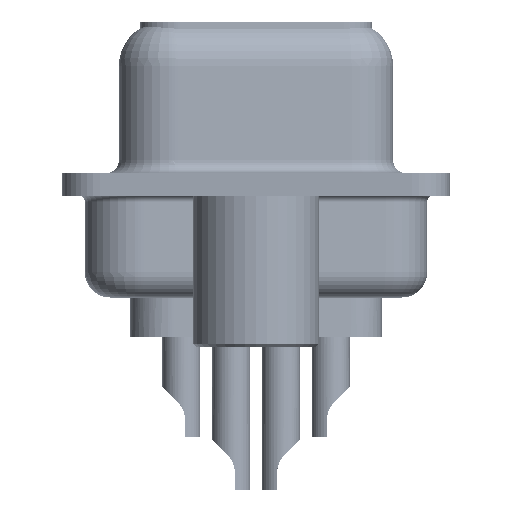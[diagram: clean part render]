
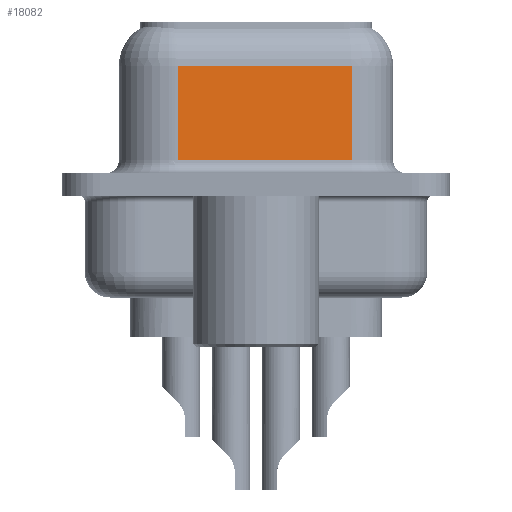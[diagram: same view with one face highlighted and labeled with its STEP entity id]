
A CAD part, left-side view. The second image highlights one B-rep face of the part: STEP entity #18082.
In plain terms, the highlighted planar face has unit normal (-0.985, -0.174, 0).
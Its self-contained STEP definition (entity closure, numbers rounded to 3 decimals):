
#115 = VECTOR ( 'NONE', #39264, 1000. ) ;
#1196 = CARTESIAN_POINT ( 'NONE',  ( 4.48, 3.103, 6.45 ) ) ;
#1555 = DIRECTION ( 'NONE',  ( 0.985, 0.174, 0. ) ) ;
#2075 = FACE_OUTER_BOUND ( 'NONE', #33271, .T. ) ;
#3596 = ORIENTED_EDGE ( 'NONE', *, *, #12378, .T. ) ;
#7317 = AXIS2_PLACEMENT_3D ( 'NONE', #17428, #1555, #42859 ) ;
#7778 = VECTOR ( 'NONE', #14341, 1000. ) ;
#8014 = CARTESIAN_POINT ( 'NONE',  ( 4.48, 3.103, 0.95 ) ) ;
#11153 = DIRECTION ( 'NONE',  ( 0., 0., -1. ) ) ;
#12378 = EDGE_CURVE ( 'NONE', #34370, #30945, #21905, .T. ) ;
#14341 = DIRECTION ( 'NONE',  ( 0.174, -0.985, 0. ) ) ;
#15179 = LINE ( 'NONE', #44382, #25253 ) ;
#16941 = EDGE_CURVE ( 'NONE', #46074, #30945, #15179, .T. ) ;
#17428 = CARTESIAN_POINT ( 'NONE',  ( 5.697, -3.797, 6.45 ) ) ;
#18082 = ADVANCED_FACE ( 'NONE', ( #2075 ), #42325, .F. ) ;
#20609 = DIRECTION ( 'NONE',  ( 0., 0., -1. ) ) ;
#21683 = LINE ( 'NONE', #1196, #40961 ) ;
#21905 = LINE ( 'NONE', #46785, #7778 ) ;
#22273 = LINE ( 'NONE', #30886, #115 ) ;
#25253 = VECTOR ( 'NONE', #11153, 1000. ) ;
#29576 = CARTESIAN_POINT ( 'NONE',  ( 5.697, -3.797, 4.7 ) ) ;
#30886 = CARTESIAN_POINT ( 'NONE',  ( 5.697, -3.797, 4.7 ) ) ;
#30945 = VERTEX_POINT ( 'NONE', #37774 ) ;
#32789 = ORIENTED_EDGE ( 'NONE', *, *, #43754, .T. ) ;
#33271 = EDGE_LOOP ( 'NONE', ( #52890, #32789, #50939, #3596 ) ) ;
#34370 = VERTEX_POINT ( 'NONE', #8014 ) ;
#37774 = CARTESIAN_POINT ( 'NONE',  ( 5.697, -3.797, 0.95 ) ) ;
#37810 = EDGE_CURVE ( 'NONE', #46921, #34370, #21683, .T. ) ;
#39264 = DIRECTION ( 'NONE',  ( -0.174, 0.985, 0. ) ) ;
#40961 = VECTOR ( 'NONE', #20609, 1000. ) ;
#42325 = PLANE ( 'NONE',  #7317 ) ;
#42859 = DIRECTION ( 'NONE',  ( -0.174, 0.985, 0. ) ) ;
#43754 = EDGE_CURVE ( 'NONE', #46074, #46921, #22273, .T. ) ;
#44382 = CARTESIAN_POINT ( 'NONE',  ( 5.697, -3.797, 6.45 ) ) ;
#46074 = VERTEX_POINT ( 'NONE', #29576 ) ;
#46424 = CARTESIAN_POINT ( 'NONE',  ( 4.48, 3.103, 4.7 ) ) ;
#46785 = CARTESIAN_POINT ( 'NONE',  ( 5.697, -3.797, 0.95 ) ) ;
#46921 = VERTEX_POINT ( 'NONE', #46424 ) ;
#50939 = ORIENTED_EDGE ( 'NONE', *, *, #37810, .T. ) ;
#52890 = ORIENTED_EDGE ( 'NONE', *, *, #16941, .F. ) ;
